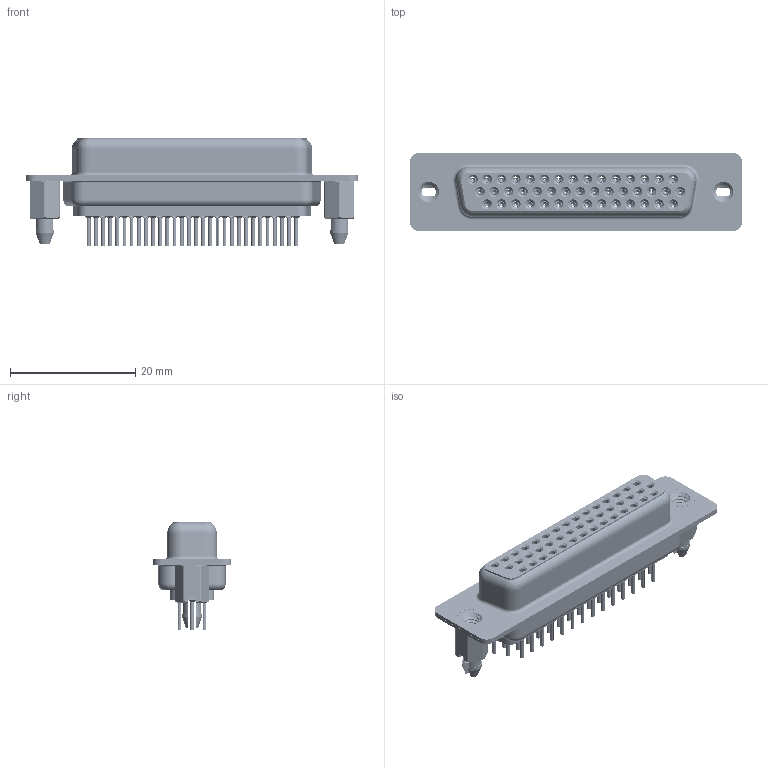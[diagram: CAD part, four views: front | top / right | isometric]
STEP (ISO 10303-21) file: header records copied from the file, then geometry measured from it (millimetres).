
FILE_DESCRIPTION (( 'STEP AP203' ), '1' );
FILE_NAME ('638-044-230-066.STEP', '2020-07-18T22:05:20', ( '' ), ( '' ), 'SwSTEP 2.0', 'SolidWorks 2020', '' );
FILE_SCHEMA (( 'CONFIG_CONTROL_DESIGN' ));
Length unit declared in the file: millimetre
Products named in the file (8): 638 Shell Rear_44 Contacts; 638 Shell Front_44 Contacts; 638 Contact Row 2_30; 638 4-40 Threaded Boardlock_LP; 638 Housing_44 Contacts; 638 Contact Row 3_30; 638 Contact Row 1_30; 638-044-230-066
Assembly tree (49 placements, depth 2):
  638-044-230-066
    638 Housing_44 Contacts
    638 Shell Front_44 Contacts
    638 Shell Rear_44 Contacts
    638 Contact Row 1_30  x15
    638 Contact Row 2_30  x15
    638 Contact Row 3_30  x14
    638 4-40 Threaded Boardlock_LP  x2
Bounding box: 53.04 x 12.6 x 17.3 mm (x, y, z)
Volume: 3376.8 mm3; surface area: 13036.8 mm2
Topology: 49 solids, 49 shells, 5941 faces, 15173 edges, 9427 vertices
Faces by surface type: cylinder 1621, plane 1463, torus 1201, bspline 886, cone 770
Entity records: 40980 total; most frequent: CARTESIAN_POINT 10977, DIRECTION 6179, ORIENTED_EDGE 5650, EDGE_CURVE 2825, AXIS2_PLACEMENT_3D 2591, VERTEX_POINT 1788, EDGE_LOOP 1433, CIRCLE 1411
